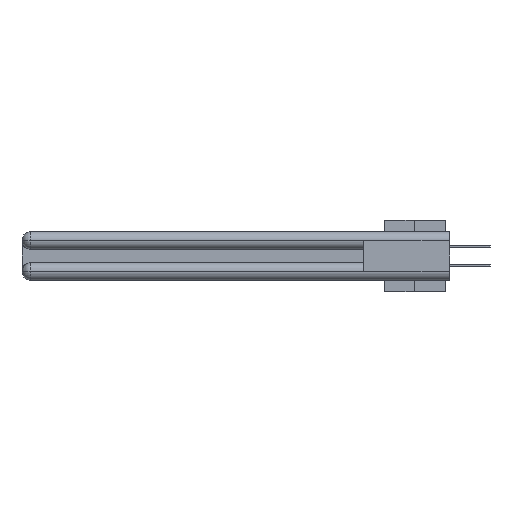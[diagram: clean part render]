
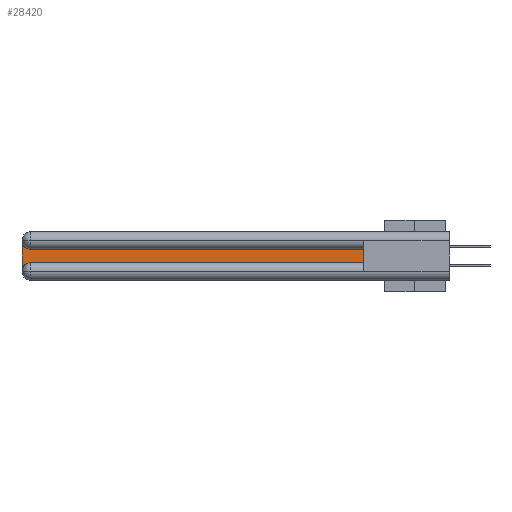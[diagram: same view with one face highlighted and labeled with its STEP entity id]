
A CAD part, left-side view. The second image highlights one B-rep face of the part: STEP entity #28420.
In plain terms, the highlighted planar face has unit normal (-1, 0, 0).
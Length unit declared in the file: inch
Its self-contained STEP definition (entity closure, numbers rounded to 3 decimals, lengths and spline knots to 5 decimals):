
#2529 = ORIENTED_EDGE ( 'NONE', *, *, #37412, .T. ) ;
#2537 = DIRECTION ( 'NONE',  ( 1., 0., 0. ) ) ;
#2856 = VERTEX_POINT ( 'NONE', #19689 ) ;
#3654 = VERTEX_POINT ( 'NONE', #8823 ) ;
#4855 = CARTESIAN_POINT ( 'NONE',  ( 0.075, 3., -0.0625 ) ) ;
#5240 = CARTESIAN_POINT ( 'NONE',  ( 0.075, 2.94, -0.0625 ) ) ;
#5351 = PLANE ( 'NONE',  #27346 ) ;
#5618 = VERTEX_POINT ( 'NONE', #25713 ) ;
#6062 = EDGE_CURVE ( 'NONE', #3654, #36501, #9341, .T. ) ;
#6294 = LINE ( 'NONE', #30032, #18162 ) ;
#7119 = LINE ( 'NONE', #22488, #37030 ) ;
#8507 = DIRECTION ( 'NONE',  ( 0., 0., -1. ) ) ;
#8823 = CARTESIAN_POINT ( 'NONE',  ( 0.075, 3., -0.2775 ) ) ;
#9341 = CIRCLE ( 'NONE', #34180, 0.06 ) ;
#10378 = DIRECTION ( 'NONE',  ( 0., -1., 0. ) ) ;
#11013 = DIRECTION ( 'NONE',  ( 0., 0., -1. ) ) ;
#11520 = EDGE_CURVE ( 'NONE', #14506, #5618, #6294, .T. ) ;
#12406 = VERTEX_POINT ( 'NONE', #4855 ) ;
#13934 = CARTESIAN_POINT ( 'NONE',  ( 0.075, 3., -0.1225 ) ) ;
#14012 = ORIENTED_EDGE ( 'NONE', *, *, #21277, .T. ) ;
#14506 = VERTEX_POINT ( 'NONE', #16974 ) ;
#14984 = DIRECTION ( 'NONE',  ( 0., 0., 1. ) ) ;
#15344 = CARTESIAN_POINT ( 'NONE',  ( 0.075, 0.6, -0.2175 ) ) ;
#15568 = LINE ( 'NONE', #28775, #17446 ) ;
#16044 = VECTOR ( 'NONE', #14984, 39.37008 ) ;
#16363 = EDGE_CURVE ( 'NONE', #12406, #3654, #7119, .T. ) ;
#16744 = AXIS2_PLACEMENT_3D ( 'NONE', #5240, #19516, #37166 ) ;
#16974 = CARTESIAN_POINT ( 'NONE',  ( 0.075, 0.6, -0.1225 ) ) ;
#17446 = VECTOR ( 'NONE', #10378, 39.37008 ) ;
#17696 = CARTESIAN_POINT ( 'NONE',  ( 0.075, 2.94, -0.2775 ) ) ;
#18162 = VECTOR ( 'NONE', #27287, 39.37008 ) ;
#19516 = DIRECTION ( 'NONE',  ( 1., 0., 0. ) ) ;
#19689 = CARTESIAN_POINT ( 'NONE',  ( 0.075, 0.6, -0.2175 ) ) ;
#20558 = FACE_OUTER_BOUND ( 'NONE', #34358, .T. ) ;
#20889 = EDGE_CURVE ( 'NONE', #2856, #14506, #22840, .T. ) ;
#21277 = EDGE_CURVE ( 'NONE', #5618, #12406, #23265, .T. ) ;
#22204 = ORIENTED_EDGE ( 'NONE', *, *, #20889, .T. ) ;
#22488 = CARTESIAN_POINT ( 'NONE',  ( 0.075, 3., -0.2175 ) ) ;
#22840 = LINE ( 'NONE', #15344, #16044 ) ;
#23265 = CIRCLE ( 'NONE', #16744, 0.06 ) ;
#25684 = DIRECTION ( 'NONE',  ( 1., 0., 0. ) ) ;
#25713 = CARTESIAN_POINT ( 'NONE',  ( 0.075, 2.94, -0.1225 ) ) ;
#27287 = DIRECTION ( 'NONE',  ( 0., 1., 0. ) ) ;
#27346 = AXIS2_PLACEMENT_3D ( 'NONE', #13934, #25684, #34398 ) ;
#28420 = ADVANCED_FACE ( 'NONE', ( #20558 ), #5351, .F. ) ;
#28775 = CARTESIAN_POINT ( 'NONE',  ( 0.075, 0.6, -0.2175 ) ) ;
#28788 = ORIENTED_EDGE ( 'NONE', *, *, #11520, .T. ) ;
#29220 = CARTESIAN_POINT ( 'NONE',  ( 0.075, 2.94, -0.2175 ) ) ;
#30032 = CARTESIAN_POINT ( 'NONE',  ( 0.075, 0.6, -0.1225 ) ) ;
#32316 = ORIENTED_EDGE ( 'NONE', *, *, #6062, .T. ) ;
#34180 = AXIS2_PLACEMENT_3D ( 'NONE', #17696, #2537, #8507 ) ;
#34358 = EDGE_LOOP ( 'NONE', ( #28788, #14012, #37158, #32316, #2529, #22204 ) ) ;
#34398 = DIRECTION ( 'NONE',  ( 0., 0., -1. ) ) ;
#36501 = VERTEX_POINT ( 'NONE', #29220 ) ;
#37030 = VECTOR ( 'NONE', #11013, 39.37008 ) ;
#37158 = ORIENTED_EDGE ( 'NONE', *, *, #16363, .T. ) ;
#37166 = DIRECTION ( 'NONE',  ( 0., 0., -1. ) ) ;
#37412 = EDGE_CURVE ( 'NONE', #36501, #2856, #15568, .T. ) ;
